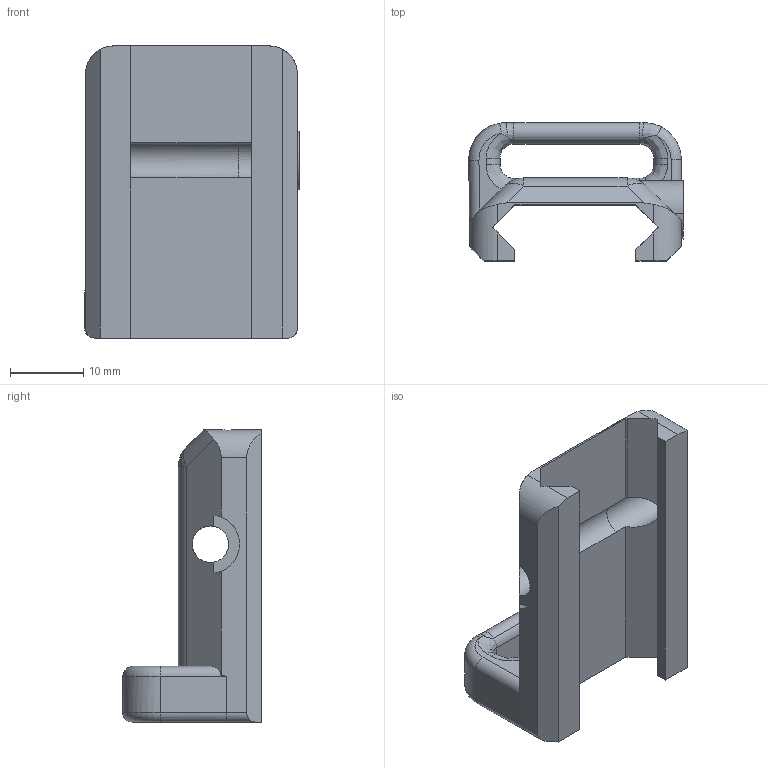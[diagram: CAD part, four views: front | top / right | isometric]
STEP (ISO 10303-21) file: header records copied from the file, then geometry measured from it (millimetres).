
FILE_DESCRIPTION(/* description */ (''),/* implementation_level */ '2;1');
FILE_NAME(/* name */ 'SG22 Sling Mount Release.step',/* time_stamp */ '2021-03-18T08:57:58-06:00',/* author */ (''),/* organization */ (''),/* preprocessor_version */ 'ST-DEVELOPER v18.1',/* originating_system */ 'Autodesk Translation Framework v9.10.0.1330',/* authorisation */ '');
FILE_SCHEMA (('AUTOMOTIVE_DESIGN { 1 0 10303 214 3 1 1 }'));
Length unit declared in the file: millimetre
Products named in the file (1): Brace V2
Bounding box: 29.38 x 18.98 x 40 mm (x, y, z)
Volume: 6465.8 mm3; surface area: 4679.9 mm2
Topology: 1 solids, 1 shells, 94 faces, 253 edges, 156 vertices
Faces by surface type: plane 37, cylinder 34, bspline 17, torus 4, sphere 2
Full cylindrical faces by diameter (mm): 5 x1, 5.045 x1
Entity records: 3567 total; most frequent: CARTESIAN_POINT 1216, ORIENTED_EDGE 506, DIRECTION 459, EDGE_CURVE 253, AXIS2_PLACEMENT_3D 171, VERTEX_POINT 156, LINE 117, VECTOR 117
